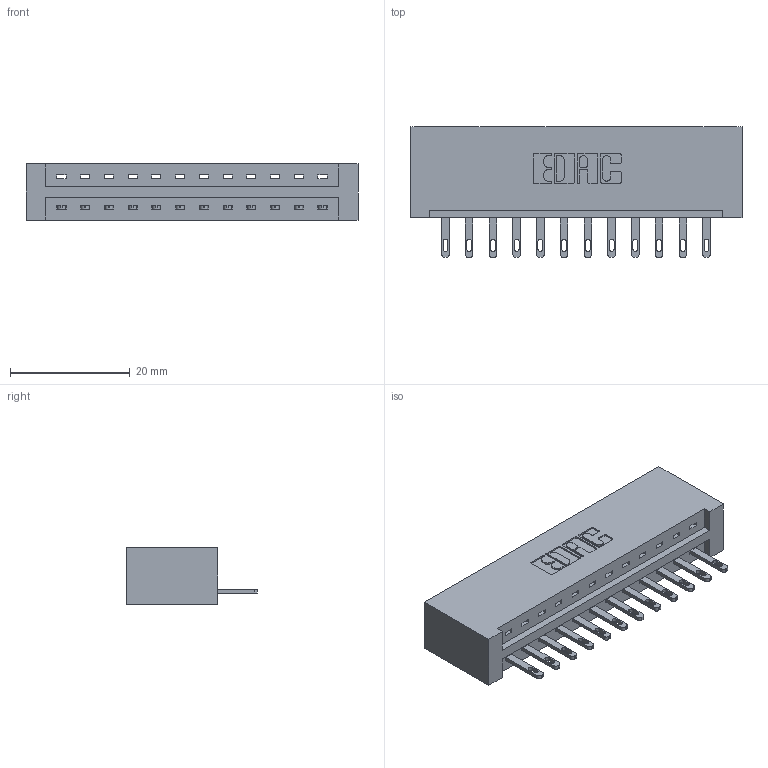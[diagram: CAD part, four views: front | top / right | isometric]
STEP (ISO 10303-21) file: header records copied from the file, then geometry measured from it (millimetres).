
FILE_DESCRIPTION (( 'STEP AP203' ), '1' );
FILE_NAME ('337-012-500-101.STEP', '2019-09-27T23:34:06', ( '' ), ( '' ), 'SwSTEP 2.0', 'SolidWorks 2016', '' );
FILE_SCHEMA (( 'CONFIG_CONTROL_DESIGN' ));
Length unit declared in the file: inch
Products named in the file (3): 337 Part_No Mounting Lugs; 337-012-500-101; 345-292-001_345-293-100
Assembly tree (13 placements, depth 2):
  337-012-500-101
    337 Part_No Mounting Lugs
    345-292-001_345-293-100  x12
Bounding box: 55.42 x 21.85 x 9.4 mm (x, y, z)
Volume: 6131 mm3; surface area: 6178.4 mm2
Topology: 13 solids, 13 shells, 802 faces, 2447 edges, 1630 vertices
Faces by surface type: plane 546, cylinder 256
Entity records: 12453 total; most frequent: CARTESIAN_POINT 2174, ORIENTED_EDGE 2122, DIRECTION 1885, EDGE_CURVE 1061, LINE 937, VECTOR 937, VERTEX_POINT 706, AXIS2_PLACEMENT_3D 474
